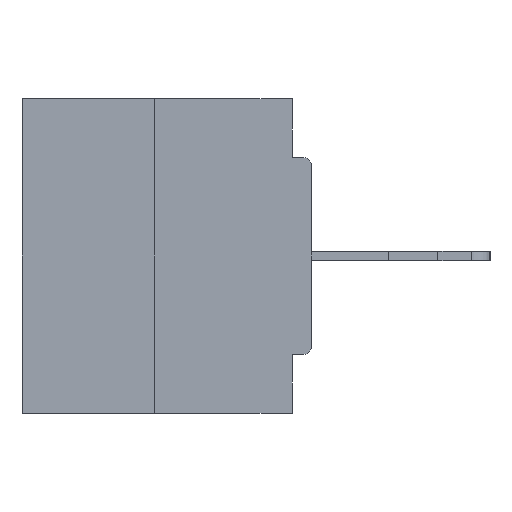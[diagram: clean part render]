
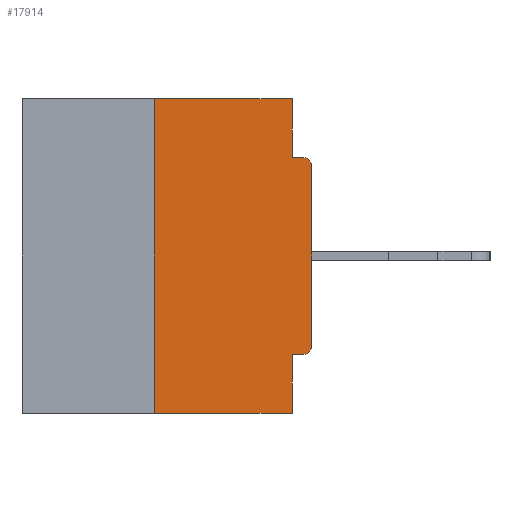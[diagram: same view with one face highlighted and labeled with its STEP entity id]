
A CAD part, left-side view. The second image highlights one B-rep face of the part: STEP entity #17914.
In plain terms, the highlighted planar face has unit normal (-1, 0, 0).
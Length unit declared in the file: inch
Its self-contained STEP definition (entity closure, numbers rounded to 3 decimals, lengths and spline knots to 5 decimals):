
#156 = CARTESIAN_POINT ( 'NONE',  ( 0., 0.031, -0.4065 ) ) ;
#244 = CIRCLE ( 'NONE', #18827, 0.015 ) ;
#392 = ORIENTED_EDGE ( 'NONE', *, *, #23654, .F. ) ;
#1002 = EDGE_CURVE ( 'NONE', #24110, #1394, #12286, .T. ) ;
#1182 = DIRECTION ( 'NONE',  ( 0., 0., -1. ) ) ;
#1394 = VERTEX_POINT ( 'NONE', #7594 ) ;
#1747 = VERTEX_POINT ( 'NONE', #23685 ) ;
#2166 = DIRECTION ( 'NONE',  ( 0., 0., -1. ) ) ;
#2492 = VECTOR ( 'NONE', #12139, 39.37008 ) ;
#3318 = DIRECTION ( 'NONE',  ( 1., 0., 0. ) ) ;
#3548 = VERTEX_POINT ( 'NONE', #15441 ) ;
#3645 = LINE ( 'NONE', #10201, #18830 ) ;
#3890 = ORIENTED_EDGE ( 'NONE', *, *, #22466, .T. ) ;
#4120 = VERTEX_POINT ( 'NONE', #9029 ) ;
#4236 = DIRECTION ( 'NONE',  ( 0., 0., -1. ) ) ;
#4247 = ORIENTED_EDGE ( 'NONE', *, *, #24969, .F. ) ;
#4300 = DIRECTION ( 'NONE',  ( 0., 0., -1. ) ) ;
#4312 = EDGE_LOOP ( 'NONE', ( #21129, #4247, #18530, #14108, #392, #14236, #10450, #3890, #4316, #13711 ) ) ;
#4316 = ORIENTED_EDGE ( 'NONE', *, *, #1002, .F. ) ;
#4442 = DIRECTION ( 'NONE',  ( -1., 0., 0. ) ) ;
#4512 = CARTESIAN_POINT ( 'NONE',  ( 0., 0.25, 0. ) ) ;
#4644 = DIRECTION ( 'NONE',  ( 0., 0., 1. ) ) ;
#4864 = CARTESIAN_POINT ( 'NONE',  ( 0., 0., -0.3915 ) ) ;
#5123 = CARTESIAN_POINT ( 'NONE',  ( 0., 0., -0.4065 ) ) ;
#5331 = FACE_OUTER_BOUND ( 'NONE', #4312, .T. ) ;
#6812 = CARTESIAN_POINT ( 'NONE',  ( 0., 0.031, -0.0935 ) ) ;
#6937 = EDGE_CURVE ( 'NONE', #3548, #8433, #244, .T. ) ;
#7031 = VECTOR ( 'NONE', #12251, 39.37008 ) ;
#7594 = CARTESIAN_POINT ( 'NONE',  ( 0., 0.015, -0.0935 ) ) ;
#7826 = LINE ( 'NONE', #16484, #7031 ) ;
#8058 = DIRECTION ( 'NONE',  ( 0., 0., 1. ) ) ;
#8433 = VERTEX_POINT ( 'NONE', #4864 ) ;
#8546 = CIRCLE ( 'NONE', #16682, 0.015 ) ;
#8568 = VECTOR ( 'NONE', #2166, 39.37008 ) ;
#8794 = CARTESIAN_POINT ( 'NONE',  ( 0., 0.031, 0. ) ) ;
#9029 = CARTESIAN_POINT ( 'NONE',  ( 0., 0.031, -0.5 ) ) ;
#9120 = CARTESIAN_POINT ( 'NONE',  ( 0., 0.46, 0. ) ) ;
#9965 = VECTOR ( 'NONE', #17895, 39.37008 ) ;
#10201 = CARTESIAN_POINT ( 'NONE',  ( 0., 0., 0. ) ) ;
#10450 = ORIENTED_EDGE ( 'NONE', *, *, #17557, .T. ) ;
#10853 = CARTESIAN_POINT ( 'NONE',  ( 0., 0.015, -0.3915 ) ) ;
#11052 = DIRECTION ( 'NONE',  ( -1., 0., 0. ) ) ;
#11295 = DIRECTION ( 'NONE',  ( 0., -1., 0. ) ) ;
#11772 = VECTOR ( 'NONE', #11295, 39.37008 ) ;
#12139 = DIRECTION ( 'NONE',  ( 0., -1., 0. ) ) ;
#12251 = DIRECTION ( 'NONE',  ( 0., 0., -1. ) ) ;
#12286 = LINE ( 'NONE', #16668, #2492 ) ;
#12684 = LINE ( 'NONE', #26017, #8568 ) ;
#12912 = CARTESIAN_POINT ( 'NONE',  ( 0., 0.015, -0.1085 ) ) ;
#13711 = ORIENTED_EDGE ( 'NONE', *, *, #20110, .F. ) ;
#14108 = ORIENTED_EDGE ( 'NONE', *, *, #23393, .F. ) ;
#14116 = PLANE ( 'NONE',  #20622 ) ;
#14236 = ORIENTED_EDGE ( 'NONE', *, *, #6937, .T. ) ;
#15441 = CARTESIAN_POINT ( 'NONE',  ( 0., 0.015, -0.4065 ) ) ;
#15899 = LINE ( 'NONE', #5123, #9965 ) ;
#16484 = CARTESIAN_POINT ( 'NONE',  ( 0., 0.031, 0. ) ) ;
#16668 = CARTESIAN_POINT ( 'NONE',  ( 0., 0., -0.0935 ) ) ;
#16682 = AXIS2_PLACEMENT_3D ( 'NONE', #12912, #11052, #4236 ) ;
#17268 = VERTEX_POINT ( 'NONE', #8794 ) ;
#17557 = EDGE_CURVE ( 'NONE', #8433, #1747, #3645, .T. ) ;
#17617 = DIRECTION ( 'NONE',  ( 0., -1., 0. ) ) ;
#17884 = LINE ( 'NONE', #9120, #24289 ) ;
#17895 = DIRECTION ( 'NONE',  ( 0., 1., 0. ) ) ;
#17914 = ADVANCED_FACE ( 'NONE', ( #5331 ), #14116, .F. ) ;
#17933 = CARTESIAN_POINT ( 'NONE',  ( 0., 0.25, -0.5 ) ) ;
#18530 = ORIENTED_EDGE ( 'NONE', *, *, #27130, .T. ) ;
#18827 = AXIS2_PLACEMENT_3D ( 'NONE', #10853, #4442, #4300 ) ;
#18830 = VECTOR ( 'NONE', #8058, 39.37008 ) ;
#19930 = CARTESIAN_POINT ( 'NONE',  ( 0., 0.25, 0. ) ) ;
#20110 = EDGE_CURVE ( 'NONE', #17268, #24110, #7826, .T. ) ;
#20470 = EDGE_CURVE ( 'NONE', #24978, #17268, #17884, .T. ) ;
#20622 = AXIS2_PLACEMENT_3D ( 'NONE', #22774, #3318, #1182 ) ;
#21129 = ORIENTED_EDGE ( 'NONE', *, *, #20470, .F. ) ;
#21235 = LINE ( 'NONE', #24193, #11772 ) ;
#21780 = VERTEX_POINT ( 'NONE', #156 ) ;
#22466 = EDGE_CURVE ( 'NONE', #1747, #1394, #8546, .T. ) ;
#22681 = VECTOR ( 'NONE', #4644, 39.37008 ) ;
#22774 = CARTESIAN_POINT ( 'NONE',  ( 0., 0.46, 0. ) ) ;
#23393 = EDGE_CURVE ( 'NONE', #21780, #4120, #12684, .T. ) ;
#23654 = EDGE_CURVE ( 'NONE', #3548, #21780, #15899, .T. ) ;
#23685 = CARTESIAN_POINT ( 'NONE',  ( 0., 0., -0.1085 ) ) ;
#24110 = VERTEX_POINT ( 'NONE', #6812 ) ;
#24193 = CARTESIAN_POINT ( 'NONE',  ( 0., 0.46, -0.5 ) ) ;
#24289 = VECTOR ( 'NONE', #17617, 39.37008 ) ;
#24969 = EDGE_CURVE ( 'NONE', #27256, #24978, #26098, .T. ) ;
#24978 = VERTEX_POINT ( 'NONE', #4512 ) ;
#26017 = CARTESIAN_POINT ( 'NONE',  ( 0., 0.031, -0.5 ) ) ;
#26098 = LINE ( 'NONE', #19930, #22681 ) ;
#27130 = EDGE_CURVE ( 'NONE', #27256, #4120, #21235, .T. ) ;
#27256 = VERTEX_POINT ( 'NONE', #17933 ) ;
